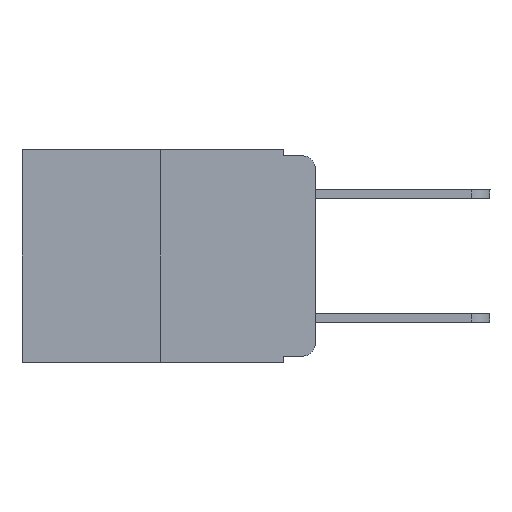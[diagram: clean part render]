
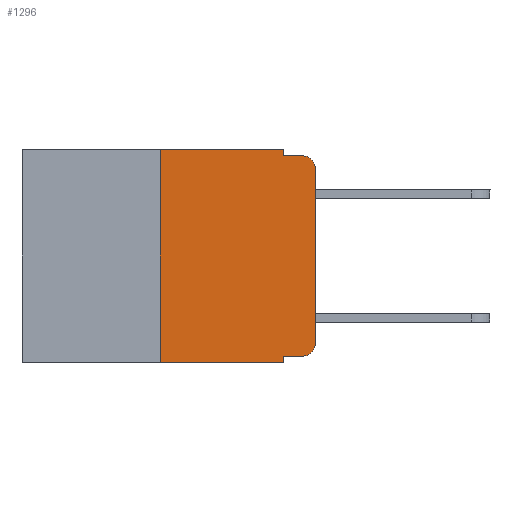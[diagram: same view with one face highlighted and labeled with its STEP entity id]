
A CAD part, left-side view. The second image highlights one B-rep face of the part: STEP entity #1296.
In plain terms, the highlighted planar face has unit normal (-1, 0, 0).
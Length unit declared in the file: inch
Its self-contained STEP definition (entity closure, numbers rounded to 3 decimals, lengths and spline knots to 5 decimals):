
#207 = FACE_OUTER_BOUND ( 'NONE', #2724, .T. ) ;
#566 = CARTESIAN_POINT ( 'NONE',  ( 0., 0.051, -0.343 ) ) ;
#593 = CARTESIAN_POINT ( 'NONE',  ( 0., 0., -0.313 ) ) ;
#657 = CARTESIAN_POINT ( 'NONE',  ( 0., 0.02, -0.313 ) ) ;
#726 = CARTESIAN_POINT ( 'NONE',  ( 0., 0.25, -0.343 ) ) ;
#808 = VERTEX_POINT ( 'NONE', #11716 ) ;
#963 = DIRECTION ( 'NONE',  ( 0., 0., -1. ) ) ;
#1081 = VECTOR ( 'NONE', #3543, 39.37008 ) ;
#1296 = ADVANCED_FACE ( 'NONE', ( #207 ), #10861, .F. ) ;
#1616 = EDGE_CURVE ( 'NONE', #1623, #7604, #12534, .T. ) ;
#1623 = VERTEX_POINT ( 'NONE', #726 ) ;
#1745 = AXIS2_PLACEMENT_3D ( 'NONE', #2036, #4122, #8086 ) ;
#1753 = EDGE_CURVE ( 'NONE', #808, #3100, #5177, .T. ) ;
#2016 = VERTEX_POINT ( 'NONE', #10685 ) ;
#2036 = CARTESIAN_POINT ( 'NONE',  ( 0., 0.473, 0. ) ) ;
#2191 = EDGE_CURVE ( 'NONE', #808, #12341, #8052, .T. ) ;
#2229 = LINE ( 'NONE', #12278, #7765 ) ;
#2313 = CIRCLE ( 'NONE', #8536, 0.02 ) ;
#2655 = ORIENTED_EDGE ( 'NONE', *, *, #10556, .T. ) ;
#2724 = EDGE_LOOP ( 'NONE', ( #6488, #11921, #3952, #3836, #12105, #12619, #8894, #10312, #6701, #2655 ) ) ;
#2825 = VERTEX_POINT ( 'NONE', #11610 ) ;
#2851 = EDGE_CURVE ( 'NONE', #11728, #7984, #2880, .T. ) ;
#2880 = LINE ( 'NONE', #6713, #9206 ) ;
#3100 = VERTEX_POINT ( 'NONE', #6436 ) ;
#3111 = DIRECTION ( 'NONE',  ( -1., 0., 0. ) ) ;
#3543 = DIRECTION ( 'NONE',  ( 0., 0., -1. ) ) ;
#3663 = DIRECTION ( 'NONE',  ( -1., 0., 0. ) ) ;
#3773 = EDGE_CURVE ( 'NONE', #9499, #2825, #9897, .T. ) ;
#3783 = CARTESIAN_POINT ( 'NONE',  ( 0., 0.25, 0. ) ) ;
#3836 = ORIENTED_EDGE ( 'NONE', *, *, #8026, .F. ) ;
#3952 = ORIENTED_EDGE ( 'NONE', *, *, #3773, .F. ) ;
#4122 = DIRECTION ( 'NONE',  ( 1., 0., 0. ) ) ;
#4856 = CARTESIAN_POINT ( 'NONE',  ( 0., 0.02, -0.03 ) ) ;
#4880 = EDGE_CURVE ( 'NONE', #7984, #2825, #2313, .T. ) ;
#4881 = DIRECTION ( 'NONE',  ( 0., 0., 1. ) ) ;
#5177 = LINE ( 'NONE', #9231, #11175 ) ;
#5450 = CARTESIAN_POINT ( 'NONE',  ( 0., 0.25, 0. ) ) ;
#5866 = EDGE_CURVE ( 'NONE', #7604, #2016, #7045, .T. ) ;
#6117 = DIRECTION ( 'NONE',  ( 0., -1., 0. ) ) ;
#6181 = DIRECTION ( 'NONE',  ( 0., -1., 0. ) ) ;
#6436 = CARTESIAN_POINT ( 'NONE',  ( 0., 0.02, -0.333 ) ) ;
#6488 = ORIENTED_EDGE ( 'NONE', *, *, #2851, .T. ) ;
#6701 = ORIENTED_EDGE ( 'NONE', *, *, #1753, .T. ) ;
#6713 = CARTESIAN_POINT ( 'NONE',  ( 0., 0., 0. ) ) ;
#6834 = DIRECTION ( 'NONE',  ( 0., 0., 1. ) ) ;
#7045 = LINE ( 'NONE', #8995, #7318 ) ;
#7318 = VECTOR ( 'NONE', #6117, 39.37008 ) ;
#7442 = CARTESIAN_POINT ( 'NONE',  ( 0., 0., -0.03 ) ) ;
#7604 = VERTEX_POINT ( 'NONE', #5450 ) ;
#7652 = CARTESIAN_POINT ( 'NONE',  ( 0., 0.051, -0.01 ) ) ;
#7765 = VECTOR ( 'NONE', #6181, 39.37008 ) ;
#7984 = VERTEX_POINT ( 'NONE', #7442 ) ;
#8026 = EDGE_CURVE ( 'NONE', #2016, #9499, #11505, .T. ) ;
#8052 = LINE ( 'NONE', #12041, #10653 ) ;
#8086 = DIRECTION ( 'NONE',  ( 0., 0., -1. ) ) ;
#8508 = VECTOR ( 'NONE', #8930, 39.37008 ) ;
#8536 = AXIS2_PLACEMENT_3D ( 'NONE', #4856, #3111, #963 ) ;
#8894 = ORIENTED_EDGE ( 'NONE', *, *, #9076, .T. ) ;
#8930 = DIRECTION ( 'NONE',  ( 0., -1., 0. ) ) ;
#8995 = CARTESIAN_POINT ( 'NONE',  ( 0., 0.473, 0. ) ) ;
#9076 = EDGE_CURVE ( 'NONE', #1623, #12341, #2229, .T. ) ;
#9206 = VECTOR ( 'NONE', #4881, 39.37008 ) ;
#9231 = CARTESIAN_POINT ( 'NONE',  ( 0., 0.051, -0.333 ) ) ;
#9499 = VERTEX_POINT ( 'NONE', #7652 ) ;
#9897 = LINE ( 'NONE', #12613, #8508 ) ;
#10108 = DIRECTION ( 'NONE',  ( 0., -1., 0. ) ) ;
#10312 = ORIENTED_EDGE ( 'NONE', *, *, #2191, .F. ) ;
#10335 = VECTOR ( 'NONE', #6834, 39.37008 ) ;
#10405 = CARTESIAN_POINT ( 'NONE',  ( 0., 0.051, 0. ) ) ;
#10556 = EDGE_CURVE ( 'NONE', #3100, #11728, #11812, .T. ) ;
#10653 = VECTOR ( 'NONE', #11178, 39.37008 ) ;
#10685 = CARTESIAN_POINT ( 'NONE',  ( 0., 0.051, 0. ) ) ;
#10770 = AXIS2_PLACEMENT_3D ( 'NONE', #657, #3663, #11547 ) ;
#10861 = PLANE ( 'NONE',  #1745 ) ;
#11175 = VECTOR ( 'NONE', #10108, 39.37008 ) ;
#11178 = DIRECTION ( 'NONE',  ( 0., 0., -1. ) ) ;
#11505 = LINE ( 'NONE', #10405, #1081 ) ;
#11547 = DIRECTION ( 'NONE',  ( 0., 0., -1. ) ) ;
#11610 = CARTESIAN_POINT ( 'NONE',  ( 0., 0.02, -0.01 ) ) ;
#11716 = CARTESIAN_POINT ( 'NONE',  ( 0., 0.051, -0.333 ) ) ;
#11728 = VERTEX_POINT ( 'NONE', #593 ) ;
#11812 = CIRCLE ( 'NONE', #10770, 0.02 ) ;
#11921 = ORIENTED_EDGE ( 'NONE', *, *, #4880, .T. ) ;
#12041 = CARTESIAN_POINT ( 'NONE',  ( 0., 0.051, 0. ) ) ;
#12105 = ORIENTED_EDGE ( 'NONE', *, *, #5866, .F. ) ;
#12278 = CARTESIAN_POINT ( 'NONE',  ( 0., 0.473, -0.343 ) ) ;
#12341 = VERTEX_POINT ( 'NONE', #566 ) ;
#12534 = LINE ( 'NONE', #3783, #10335 ) ;
#12613 = CARTESIAN_POINT ( 'NONE',  ( 0., 0.051, -0.01 ) ) ;
#12619 = ORIENTED_EDGE ( 'NONE', *, *, #1616, .F. ) ;
